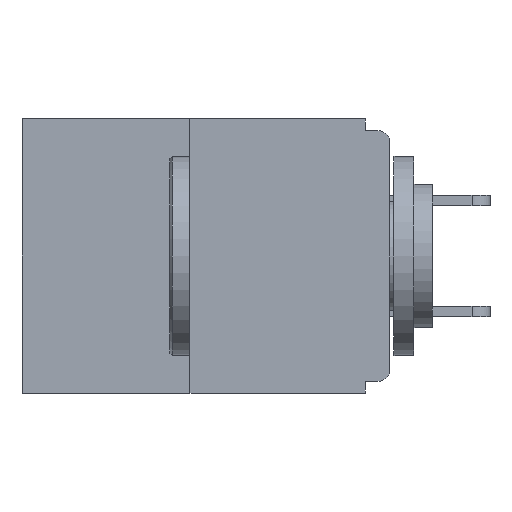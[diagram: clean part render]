
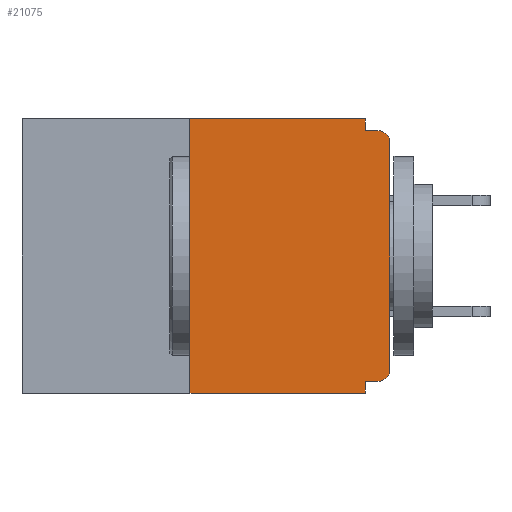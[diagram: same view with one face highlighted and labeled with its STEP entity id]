
A CAD part, left-side view. The second image highlights one B-rep face of the part: STEP entity #21075.
In plain terms, the highlighted planar face has unit normal (-1, 0, 0).
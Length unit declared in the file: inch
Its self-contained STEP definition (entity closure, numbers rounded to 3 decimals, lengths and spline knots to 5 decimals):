
#192 = CARTESIAN_POINT ( 'NONE',  ( 0., 0.46, 0. ) ) ;
#233 = CIRCLE ( 'NONE', #4681, 0.015 ) ;
#1430 = VECTOR ( 'NONE', #6410, 39.37008 ) ;
#1458 = EDGE_CURVE ( 'NONE', #6028, #19870, #13259, .T. ) ;
#1722 = CARTESIAN_POINT ( 'NONE',  ( 0., 0., -0.015 ) ) ;
#2699 = CARTESIAN_POINT ( 'NONE',  ( 0., 0., -0.03 ) ) ;
#2946 = CARTESIAN_POINT ( 'NONE',  ( 0., 0.46, 0. ) ) ;
#3652 = CARTESIAN_POINT ( 'NONE',  ( 0., 0.031, -0.343 ) ) ;
#3742 = CARTESIAN_POINT ( 'NONE',  ( 0., 0., -0.313 ) ) ;
#4661 = DIRECTION ( 'NONE',  ( 1., 0., 0. ) ) ;
#4681 = AXIS2_PLACEMENT_3D ( 'NONE', #12327, #15916, #4957 ) ;
#4770 = CARTESIAN_POINT ( 'NONE',  ( 0., 0.25, -0.343 ) ) ;
#4957 = DIRECTION ( 'NONE',  ( 0., 0., -1. ) ) ;
#5578 = EDGE_CURVE ( 'NONE', #21609, #6028, #16726, .T. ) ;
#5763 = DIRECTION ( 'NONE',  ( 0., -1., 0. ) ) ;
#5922 = DIRECTION ( 'NONE',  ( 0., 0., -1. ) ) ;
#6028 = VERTEX_POINT ( 'NONE', #2699 ) ;
#6410 = DIRECTION ( 'NONE',  ( 0., 0., 1. ) ) ;
#6476 = VECTOR ( 'NONE', #11420, 39.37008 ) ;
#6586 = PLANE ( 'NONE',  #21686 ) ;
#7372 = CARTESIAN_POINT ( 'NONE',  ( 0., 0.031, 0. ) ) ;
#7711 = DIRECTION ( 'NONE',  ( 0., -1., 0. ) ) ;
#7801 = CARTESIAN_POINT ( 'NONE',  ( 0., 0.031, -0.328 ) ) ;
#7974 = VERTEX_POINT ( 'NONE', #12686 ) ;
#9324 = ORIENTED_EDGE ( 'NONE', *, *, #19810, .F. ) ;
#9368 = ORIENTED_EDGE ( 'NONE', *, *, #20544, .T. ) ;
#9388 = CARTESIAN_POINT ( 'NONE',  ( 0., 0., 0. ) ) ;
#9633 = EDGE_CURVE ( 'NONE', #18401, #22468, #16217, .T. ) ;
#10298 = CARTESIAN_POINT ( 'NONE',  ( 0., 0., -0.328 ) ) ;
#10391 = ORIENTED_EDGE ( 'NONE', *, *, #18158, .F. ) ;
#10573 = ORIENTED_EDGE ( 'NONE', *, *, #21986, .F. ) ;
#11420 = DIRECTION ( 'NONE',  ( 0., 0., -1. ) ) ;
#12183 = VECTOR ( 'NONE', #24281, 39.37008 ) ;
#12327 = CARTESIAN_POINT ( 'NONE',  ( 0., 0.015, -0.313 ) ) ;
#12581 = DIRECTION ( 'NONE',  ( 0., 0., -1. ) ) ;
#12686 = CARTESIAN_POINT ( 'NONE',  ( 0., 0.25, 0. ) ) ;
#12918 = VERTEX_POINT ( 'NONE', #7801 ) ;
#13230 = LINE ( 'NONE', #20766, #6476 ) ;
#13259 = CIRCLE ( 'NONE', #13640, 0.015 ) ;
#13640 = AXIS2_PLACEMENT_3D ( 'NONE', #23833, #21956, #12581 ) ;
#13675 = FACE_OUTER_BOUND ( 'NONE', #17694, .T. ) ;
#13856 = VECTOR ( 'NONE', #7711, 39.37008 ) ;
#14842 = ORIENTED_EDGE ( 'NONE', *, *, #23325, .F. ) ;
#14892 = VECTOR ( 'NONE', #21649, 39.37008 ) ;
#15524 = CARTESIAN_POINT ( 'NONE',  ( 0., 0.031, -0.343 ) ) ;
#15663 = EDGE_CURVE ( 'NONE', #7974, #21996, #16938, .T. ) ;
#15887 = VECTOR ( 'NONE', #18292, 39.37008 ) ;
#15916 = DIRECTION ( 'NONE',  ( -1., 0., 0. ) ) ;
#16217 = LINE ( 'NONE', #19184, #13856 ) ;
#16282 = LINE ( 'NONE', #1722, #12183 ) ;
#16319 = CARTESIAN_POINT ( 'NONE',  ( 0., 0.25, 0. ) ) ;
#16726 = LINE ( 'NONE', #9388, #1430 ) ;
#16938 = LINE ( 'NONE', #192, #21924 ) ;
#17694 = EDGE_LOOP ( 'NONE', ( #23830, #19955, #21355, #10391, #9324, #9368, #22628, #18364, #10573, #14842 ) ) ;
#17920 = CARTESIAN_POINT ( 'NONE',  ( 0., 0.015, -0.015 ) ) ;
#17930 = VERTEX_POINT ( 'NONE', #19689 ) ;
#18158 = EDGE_CURVE ( 'NONE', #12918, #22468, #23123, .T. ) ;
#18292 = DIRECTION ( 'NONE',  ( 0., 0., 1. ) ) ;
#18364 = ORIENTED_EDGE ( 'NONE', *, *, #1458, .T. ) ;
#18401 = VERTEX_POINT ( 'NONE', #4770 ) ;
#18944 = CARTESIAN_POINT ( 'NONE',  ( 0., 0.015, -0.328 ) ) ;
#19138 = LINE ( 'NONE', #16319, #15887 ) ;
#19184 = CARTESIAN_POINT ( 'NONE',  ( 0., 0.46, -0.343 ) ) ;
#19689 = CARTESIAN_POINT ( 'NONE',  ( 0., 0.031, -0.015 ) ) ;
#19810 = EDGE_CURVE ( 'NONE', #24167, #12918, #22245, .T. ) ;
#19870 = VERTEX_POINT ( 'NONE', #17920 ) ;
#19955 = ORIENTED_EDGE ( 'NONE', *, *, #22896, .F. ) ;
#20544 = EDGE_CURVE ( 'NONE', #24167, #21609, #233, .T. ) ;
#20766 = CARTESIAN_POINT ( 'NONE',  ( 0., 0.031, 0. ) ) ;
#21075 = ADVANCED_FACE ( 'NONE', ( #13675 ), #6586, .F. ) ;
#21119 = VECTOR ( 'NONE', #5922, 39.37008 ) ;
#21355 = ORIENTED_EDGE ( 'NONE', *, *, #9633, .T. ) ;
#21609 = VERTEX_POINT ( 'NONE', #3742 ) ;
#21642 = DIRECTION ( 'NONE',  ( 0., 0., -1. ) ) ;
#21649 = DIRECTION ( 'NONE',  ( 0., 1., 0. ) ) ;
#21686 = AXIS2_PLACEMENT_3D ( 'NONE', #2946, #4661, #21642 ) ;
#21924 = VECTOR ( 'NONE', #5763, 39.37008 ) ;
#21956 = DIRECTION ( 'NONE',  ( -1., 0., 0. ) ) ;
#21986 = EDGE_CURVE ( 'NONE', #17930, #19870, #16282, .T. ) ;
#21996 = VERTEX_POINT ( 'NONE', #7372 ) ;
#22245 = LINE ( 'NONE', #10298, #14892 ) ;
#22468 = VERTEX_POINT ( 'NONE', #15524 ) ;
#22628 = ORIENTED_EDGE ( 'NONE', *, *, #5578, .T. ) ;
#22896 = EDGE_CURVE ( 'NONE', #18401, #7974, #19138, .T. ) ;
#23123 = LINE ( 'NONE', #3652, #21119 ) ;
#23325 = EDGE_CURVE ( 'NONE', #21996, #17930, #13230, .T. ) ;
#23830 = ORIENTED_EDGE ( 'NONE', *, *, #15663, .F. ) ;
#23833 = CARTESIAN_POINT ( 'NONE',  ( 0., 0.015, -0.03 ) ) ;
#24167 = VERTEX_POINT ( 'NONE', #18944 ) ;
#24281 = DIRECTION ( 'NONE',  ( 0., -1., 0. ) ) ;
